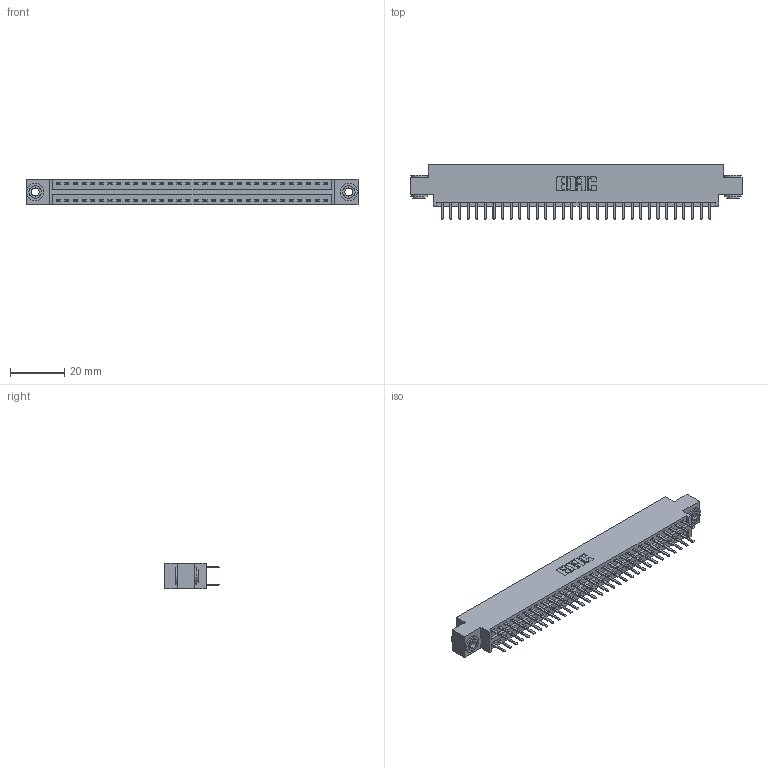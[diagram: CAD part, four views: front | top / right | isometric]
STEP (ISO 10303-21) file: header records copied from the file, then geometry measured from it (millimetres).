
FILE_DESCRIPTION (( 'STEP AP203' ), '1' );
FILE_NAME ('346-064-520-803.STEP', '2018-08-28T08:33:00', ( '' ), ( '' ), 'SwSTEP 2.0', 'SolidWorks 2016', '' );
FILE_SCHEMA (( 'CONFIG_CONTROL_DESIGN' ));
Length unit declared in the file: inch
Products named in the file (4): 345-292-001_345-293-120; 345-250-002_345-250-002-102; 346-064-520-803; 346 Part_0.170 Offset - 0.156 Dia-TH
Assembly tree (67 placements, depth 2):
  346-064-520-803
    346 Part_0.170 Offset - 0.156 Dia-TH
    345-292-001_345-293-120  x64
    345-250-002_345-250-002-102  x2
Bounding box: 122.17 x 20.02 x 9.4 mm (x, y, z)
Volume: 11672.5 mm3; surface area: 16215.3 mm2
Topology: 67 solids, 67 shells, 3748 faces, 10849 edges, 7058 vertices
Faces by surface type: plane 2458, cylinder 1282, cone 8
Entity records: 23126 total; most frequent: CARTESIAN_POINT 3815, ORIENTED_EDGE 3730, DIRECTION 3431, EDGE_CURVE 1865, VECTOR 1577, LINE 1577, VERTEX_POINT 1238, AXIS2_PLACEMENT_3D 927
